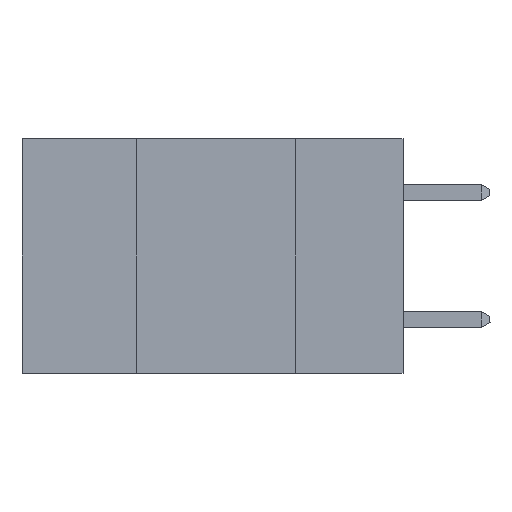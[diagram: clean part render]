
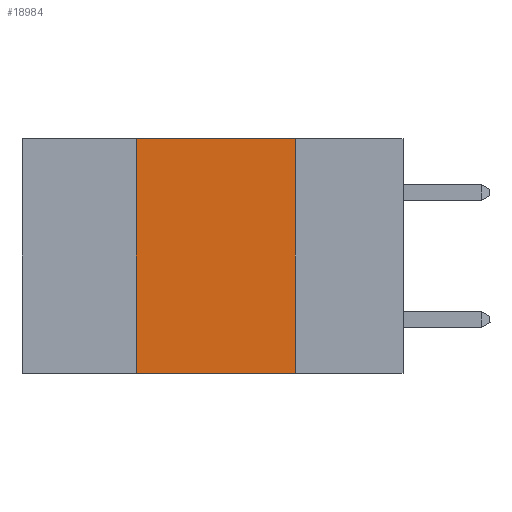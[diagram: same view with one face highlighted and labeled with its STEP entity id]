
A CAD part, left-side view. The second image highlights one B-rep face of the part: STEP entity #18984.
In plain terms, the highlighted planar face has unit normal (-1, 0, 0).
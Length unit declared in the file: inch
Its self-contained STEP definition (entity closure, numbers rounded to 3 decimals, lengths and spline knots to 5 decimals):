
#2390 = VERTEX_POINT ( 'NONE', #24359 ) ;
#4146 = DIRECTION ( 'NONE',  ( 0., 0., -1. ) ) ;
#4156 = CARTESIAN_POINT ( 'NONE',  ( 0., 0.6, 0. ) ) ;
#4458 = LINE ( 'NONE', #19790, #19268 ) ;
#4545 = AXIS2_PLACEMENT_3D ( 'NONE', #28103, #9727, #21414 ) ;
#5811 = LINE ( 'NONE', #4156, #27326 ) ;
#7418 = FACE_OUTER_BOUND ( 'NONE', #30284, .T. ) ;
#8780 = VERTEX_POINT ( 'NONE', #38271 ) ;
#9727 = DIRECTION ( 'NONE',  ( 1., 0., 0. ) ) ;
#10627 = VERTEX_POINT ( 'NONE', #30750 ) ;
#12092 = ORIENTED_EDGE ( 'NONE', *, *, #27172, .F. ) ;
#12751 = CARTESIAN_POINT ( 'NONE',  ( 0., 0.42, 0. ) ) ;
#13658 = EDGE_CURVE ( 'NONE', #10627, #32619, #23749, .T. ) ;
#14942 = ORIENTED_EDGE ( 'NONE', *, *, #24372, .F. ) ;
#15378 = PLANE ( 'NONE',  #4545 ) ;
#18984 = ADVANCED_FACE ( 'NONE', ( #7418 ), #15378, .F. ) ;
#19268 = VECTOR ( 'NONE', #4146, 39.37008 ) ;
#19790 = CARTESIAN_POINT ( 'NONE',  ( 0., 0.17, 0. ) ) ;
#20812 = LINE ( 'NONE', #12751, #38047 ) ;
#21414 = DIRECTION ( 'NONE',  ( 0., 0., -1. ) ) ;
#21524 = DIRECTION ( 'NONE',  ( 0., -1., 0. ) ) ;
#21883 = DIRECTION ( 'NONE',  ( 0., 0., 1. ) ) ;
#22102 = CARTESIAN_POINT ( 'NONE',  ( 0., 0.17, -0.37 ) ) ;
#23749 = LINE ( 'NONE', #27565, #30919 ) ;
#24359 = CARTESIAN_POINT ( 'NONE',  ( 0., 0.42, 0. ) ) ;
#24372 = EDGE_CURVE ( 'NONE', #10627, #2390, #20812, .T. ) ;
#25565 = DIRECTION ( 'NONE',  ( 0., -1., 0. ) ) ;
#25914 = EDGE_CURVE ( 'NONE', #8780, #32619, #4458, .T. ) ;
#27172 = EDGE_CURVE ( 'NONE', #2390, #8780, #5811, .T. ) ;
#27326 = VECTOR ( 'NONE', #25565, 39.37008 ) ;
#27565 = CARTESIAN_POINT ( 'NONE',  ( 0., 0.6, -0.37 ) ) ;
#28103 = CARTESIAN_POINT ( 'NONE',  ( 0., 0.6, 0. ) ) ;
#30284 = EDGE_LOOP ( 'NONE', ( #31719, #12092, #14942, #36151 ) ) ;
#30750 = CARTESIAN_POINT ( 'NONE',  ( 0., 0.42, -0.37 ) ) ;
#30919 = VECTOR ( 'NONE', #21524, 39.37008 ) ;
#31719 = ORIENTED_EDGE ( 'NONE', *, *, #25914, .F. ) ;
#32619 = VERTEX_POINT ( 'NONE', #22102 ) ;
#36151 = ORIENTED_EDGE ( 'NONE', *, *, #13658, .T. ) ;
#38047 = VECTOR ( 'NONE', #21883, 39.37008 ) ;
#38271 = CARTESIAN_POINT ( 'NONE',  ( 0., 0.17, 0. ) ) ;
